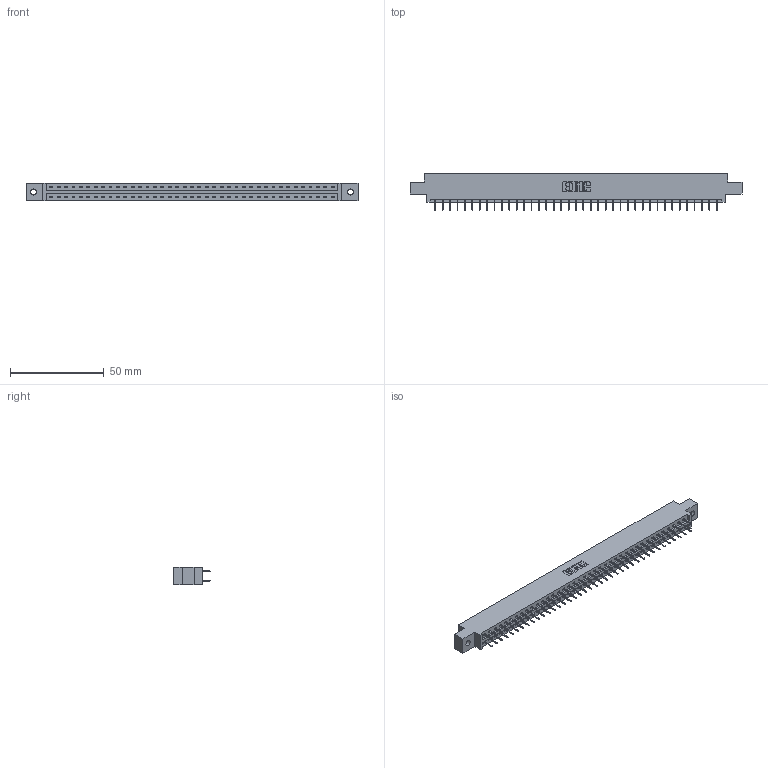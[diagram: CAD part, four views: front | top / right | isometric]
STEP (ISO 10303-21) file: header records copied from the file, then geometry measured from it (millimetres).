
FILE_DESCRIPTION (( 'STEP AP203' ), '1' );
FILE_NAME ('337-078-524-802.STEP', '2019-10-15T14:10:00', ( '' ), ( '' ), 'SwSTEP 2.0', 'SolidWorks 2016', '' );
FILE_SCHEMA (( 'CONFIG_CONTROL_DESIGN' ));
Length unit declared in the file: inch
Products named in the file (3): 337-078-524-802; 337 Part_0.170 Offset - 0.128 Dia; 345-292-001_345-293-124
Assembly tree (79 placements, depth 2):
  337-078-524-802
    337 Part_0.170 Offset - 0.128 Dia
    345-292-001_345-293-124  x78
Bounding box: 177.55 x 19.69 x 9.4 mm (x, y, z)
Volume: 18399 mm3; surface area: 20240.5 mm2
Topology: 79 solids, 79 shells, 4642 faces, 13193 edges, 8482 vertices
Faces by surface type: plane 3506, cylinder 1136
Entity records: 30835 total; most frequent: CARTESIAN_POINT 5198, ORIENTED_EDGE 5134, DIRECTION 4427, EDGE_CURVE 2567, VECTOR 2443, LINE 2443, VERTEX_POINT 1706, AXIS2_PLACEMENT_3D 992
